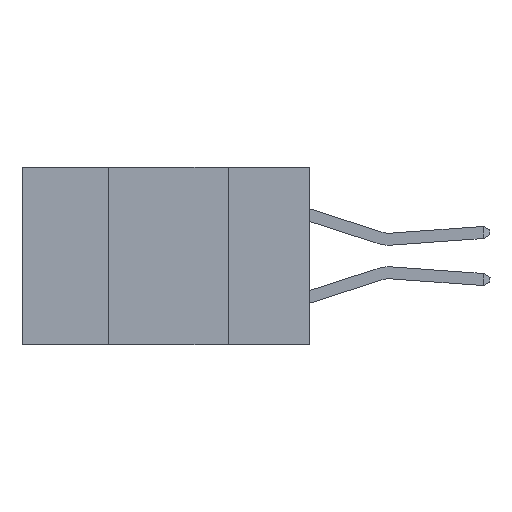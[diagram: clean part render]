
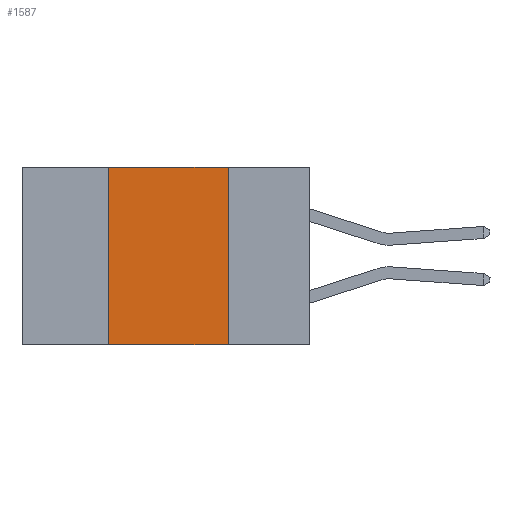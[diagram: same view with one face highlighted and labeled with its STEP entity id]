
A CAD part, left-side view. The second image highlights one B-rep face of the part: STEP entity #1587.
In plain terms, the highlighted planar face has unit normal (-1, 0, 0).
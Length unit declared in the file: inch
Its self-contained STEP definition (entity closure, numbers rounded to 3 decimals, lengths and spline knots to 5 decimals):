
#25 = DIRECTION ( 'NONE',  ( 0., 0., -1. ) ) ;
#49 = DIRECTION ( 'NONE',  ( 1., 0., 0. ) ) ;
#64 = CARTESIAN_POINT ( 'NONE',  ( 0., 0.17, 0. ) ) ;
#72 = CARTESIAN_POINT ( 'NONE',  ( 0., 0.6, 0. ) ) ;
#204 = PLANE ( 'NONE',  #10891 ) ;
#668 = EDGE_CURVE ( 'NONE', #14333, #1781, #16059, .T. ) ;
#1587 = ADVANCED_FACE ( 'NONE', ( #8356 ), #204, .F. ) ;
#1781 = VERTEX_POINT ( 'NONE', #17473 ) ;
#1900 = VERTEX_POINT ( 'NONE', #21122 ) ;
#2359 = DIRECTION ( 'NONE',  ( 0., 0., 1. ) ) ;
#2572 = LINE ( 'NONE', #20693, #16476 ) ;
#3431 = EDGE_CURVE ( 'NONE', #7973, #1781, #16391, .T. ) ;
#3958 = VECTOR ( 'NONE', #2359, 39.37008 ) ;
#4926 = CARTESIAN_POINT ( 'NONE',  ( 0., 0.6, -0.37 ) ) ;
#5037 = DIRECTION ( 'NONE',  ( 0., -1., 0. ) ) ;
#6393 = ORIENTED_EDGE ( 'NONE', *, *, #8133, .F. ) ;
#7796 = ORIENTED_EDGE ( 'NONE', *, *, #668, .F. ) ;
#7973 = VERTEX_POINT ( 'NONE', #13731 ) ;
#8060 = ORIENTED_EDGE ( 'NONE', *, *, #3431, .T. ) ;
#8133 = EDGE_CURVE ( 'NONE', #1900, #14333, #2572, .T. ) ;
#8356 = FACE_OUTER_BOUND ( 'NONE', #14847, .T. ) ;
#8771 = VECTOR ( 'NONE', #5037, 39.37008 ) ;
#10371 = EDGE_CURVE ( 'NONE', #7973, #1900, #17307, .T. ) ;
#10891 = AXIS2_PLACEMENT_3D ( 'NONE', #72, #49, #25 ) ;
#12588 = CARTESIAN_POINT ( 'NONE',  ( 0., 0.42, -0.37 ) ) ;
#13731 = CARTESIAN_POINT ( 'NONE',  ( 0., 0.42, -0.37 ) ) ;
#14140 = DIRECTION ( 'NONE',  ( 0., -1., 0. ) ) ;
#14333 = VERTEX_POINT ( 'NONE', #64 ) ;
#14847 = EDGE_LOOP ( 'NONE', ( #7796, #6393, #20177, #8060 ) ) ;
#16059 = LINE ( 'NONE', #20955, #20491 ) ;
#16391 = LINE ( 'NONE', #4926, #8771 ) ;
#16476 = VECTOR ( 'NONE', #14140, 39.37008 ) ;
#17307 = LINE ( 'NONE', #12588, #3958 ) ;
#17473 = CARTESIAN_POINT ( 'NONE',  ( 0., 0.17, -0.37 ) ) ;
#20177 = ORIENTED_EDGE ( 'NONE', *, *, #10371, .F. ) ;
#20491 = VECTOR ( 'NONE', #21469, 39.37008 ) ;
#20693 = CARTESIAN_POINT ( 'NONE',  ( 0., 0.6, 0. ) ) ;
#20955 = CARTESIAN_POINT ( 'NONE',  ( 0., 0.17, -0.37 ) ) ;
#21122 = CARTESIAN_POINT ( 'NONE',  ( 0., 0.42, 0. ) ) ;
#21469 = DIRECTION ( 'NONE',  ( 0., 0., -1. ) ) ;
